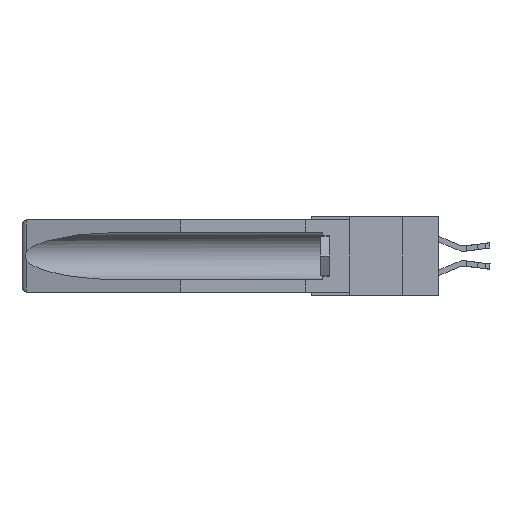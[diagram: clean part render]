
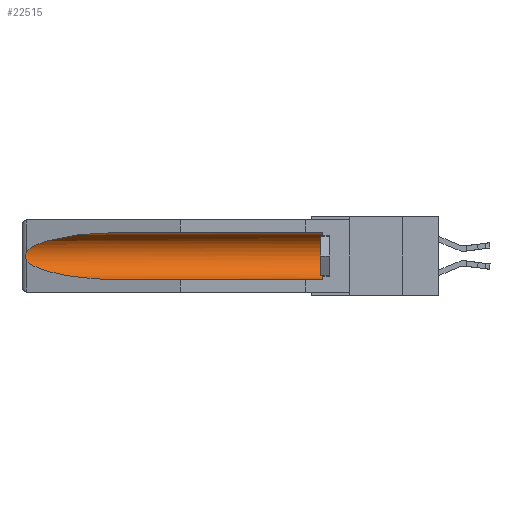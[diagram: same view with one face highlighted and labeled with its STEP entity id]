
A CAD part, left-side view. The second image highlights one B-rep face of the part: STEP entity #22515.
In plain terms, the highlighted cylindrical face has radius 2.857 mm (diameter 5.715 mm), a partial arc.
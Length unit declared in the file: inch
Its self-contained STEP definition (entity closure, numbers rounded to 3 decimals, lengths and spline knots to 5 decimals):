
#391 = CARTESIAN_POINT ( 'NONE',  ( 0.26537, 1.52718, -0.19328 ) ) ;
#412 = CARTESIAN_POINT ( 'NONE',  ( 0.155, 1.07973, -0.059 ) ) ;
#650 = ORIENTED_EDGE ( 'NONE', *, *, #18229, .T. ) ;
#932 = ORIENTED_EDGE ( 'NONE', *, *, #18708, .T. ) ;
#1380 = CARTESIAN_POINT ( 'NONE',  ( 0.25451, 1.48313, -0.24835 ) ) ;
#1624 = EDGE_CURVE ( 'NONE', #8203, #10689, #21690, .T. ) ;
#2070 = CARTESIAN_POINT ( 'NONE',  ( 0.26537, 1.52718, -0.14972 ) ) ;
#3521 = CIRCLE ( 'NONE', #14545, 0.1125 ) ;
#4706 = DIRECTION ( 'NONE',  ( 0., 1., 0. ) ) ;
#4957 = CARTESIAN_POINT ( 'NONE',  ( 0.155, 1.07973, -0.059 ) ) ;
#5436 = CARTESIAN_POINT ( 'NONE',  ( 0.2675, 1.53308, -0.16763 ) ) ;
#6120 = DIRECTION ( 'NONE',  ( 0., 1., 0. ) ) ;
#6589 = CARTESIAN_POINT ( 'NONE',  ( 0.155, 1.07973, -0.284 ) ) ;
#6967 = CARTESIAN_POINT ( 'NONE',  ( 0.2675, 1.53308, -0.17534 ) ) ;
#7113 = CARTESIAN_POINT ( 'NONE',  ( 0.26655, 1.53094, -0.18657 ) ) ;
#7624 = DIRECTION ( 'NONE',  ( 0., 0., 1. ) ) ;
#7656 = B_SPLINE_CURVE_WITH_KNOTS ( 'NONE', 3,
 ( #19102, #15642, #17405, #12399, #5436, #6967, #8620, #7113, #12183, #13880 ),
 .UNSPECIFIED., .F., .F.,
 ( 4, 2, 2, 2, 4 ),
 ( 0., 0.00029, 0.00058, 0.00087, 0.00117 ),
 .UNSPECIFIED. ) ;
#8203 = VERTEX_POINT ( 'NONE', #14624 ) ;
#8305 = CARTESIAN_POINT ( 'NONE',  ( 0.155, 1.07973, -0.284 ) ) ;
#8620 = CARTESIAN_POINT ( 'NONE',  ( 0.2673, 1.53269, -0.17917 ) ) ;
#8873 = CYLINDRICAL_SURFACE ( 'NONE', #9598, 0.1125 ) ;
#9003 = VERTEX_POINT ( 'NONE', #391 ) ;
#9062 = ORIENTED_EDGE ( 'NONE', *, *, #21922, .T. ) ;
#9598 = AXIS2_PLACEMENT_3D ( 'NONE', #14553, #10896, #7624 ) ;
#9942 = CARTESIAN_POINT ( 'NONE',  ( 0.155, -0.30754, -0.059 ) ) ;
#10052 = CARTESIAN_POINT ( 'NONE',  ( 0.25451, 1.48313, -0.09465 ) ) ;
#10334 = DIRECTION ( 'NONE',  ( 0., 0., 1. ) ) ;
#10689 = VERTEX_POINT ( 'NONE', #6589 ) ;
#10896 = DIRECTION ( 'NONE',  ( 0., 1., 0. ) ) ;
#11563 = CARTESIAN_POINT ( 'NONE',  ( 0.21114, 1.30732, -0.284 ) ) ;
#11685 = ORIENTED_EDGE ( 'NONE', *, *, #21661, .T. ) ;
#11702 = CARTESIAN_POINT ( 'NONE',  ( 0.26537, 1.52718, -0.19328 ) ) ;
#12183 = CARTESIAN_POINT ( 'NONE',  ( 0.26597, 1.5296, -0.19026 ) ) ;
#12399 = CARTESIAN_POINT ( 'NONE',  ( 0.2673, 1.5327, -0.16383 ) ) ;
#12922 = CARTESIAN_POINT ( 'NONE',  ( 0.155, -0.30754, -0.284 ) ) ;
#13310 = EDGE_CURVE ( 'NONE', #8203, #20683, #3521, .T. ) ;
#13880 = CARTESIAN_POINT ( 'NONE',  ( 0.26537, 1.52718, -0.19328 ) ) ;
#14545 = AXIS2_PLACEMENT_3D ( 'NONE', #22470, #15451, #10334 ) ;
#14553 = CARTESIAN_POINT ( 'NONE',  ( 0.155, -0.30754, -0.1715 ) ) ;
#14624 = CARTESIAN_POINT ( 'NONE',  ( 0.155, 0.126, -0.284 ) ) ;
#15451 = DIRECTION ( 'NONE',  ( 0., -1., 0. ) ) ;
#15622 = ORIENTED_EDGE ( 'NONE', *, *, #13310, .T. ) ;
#15642 = CARTESIAN_POINT ( 'NONE',  ( 0.26597, 1.52961, -0.15275 ) ) ;
#16323 = EDGE_LOOP ( 'NONE', ( #932, #650, #11685, #22556, #15622, #9062 ) ) ;
#16462 = VERTEX_POINT ( 'NONE', #2070 ) ;
#16536 = LINE ( 'NONE', #9942, #18746 ) ;
#17174 = CARTESIAN_POINT ( 'NONE',  ( 0.26537, 1.52718, -0.14972 ) ) ;
#17405 = CARTESIAN_POINT ( 'NONE',  ( 0.26654, 1.53092, -0.15636 ) ) ;
#17438 =( BOUNDED_CURVE ( )  B_SPLINE_CURVE ( 3, ( #11702, #1380, #11563, #8305 ),
 .UNSPECIFIED., .F., .F. ) 
 B_SPLINE_CURVE_WITH_KNOTS ( ( 4, 4 ),
 ( 0.1948, 1.5708 ),
 .UNSPECIFIED. ) 
 CURVE ( )  GEOMETRIC_REPRESENTATION_ITEM ( )  RATIONAL_B_SPLINE_CURVE ( ( 1., 0.848, 0.848, 1. ) ) 
 REPRESENTATION_ITEM ( '' )  );
#17898 = FACE_OUTER_BOUND ( 'NONE', #16323, .T. ) ;
#17938 = VERTEX_POINT ( 'NONE', #412 ) ;
#18229 = EDGE_CURVE ( 'NONE', #16462, #9003, #7656, .T. ) ;
#18418 = VECTOR ( 'NONE', #6120, 39.37008 ) ;
#18708 = EDGE_CURVE ( 'NONE', #17938, #16462, #19136, .T. ) ;
#18746 = VECTOR ( 'NONE', #4706, 39.37008 ) ;
#19102 = CARTESIAN_POINT ( 'NONE',  ( 0.26537, 1.52718, -0.14972 ) ) ;
#19136 =( BOUNDED_CURVE ( )  B_SPLINE_CURVE ( 3, ( #4957, #20525, #10052, #17174 ),
 .UNSPECIFIED., .F., .T. ) 
 B_SPLINE_CURVE_WITH_KNOTS ( ( 4, 4 ),
 ( 4.71239, 6.08839 ),
 .UNSPECIFIED. ) 
 CURVE ( )  GEOMETRIC_REPRESENTATION_ITEM ( )  RATIONAL_B_SPLINE_CURVE ( ( 1., 0.848, 0.848, 1. ) ) 
 REPRESENTATION_ITEM ( '' )  );
#20525 = CARTESIAN_POINT ( 'NONE',  ( 0.21114, 1.30732, -0.059 ) ) ;
#20683 = VERTEX_POINT ( 'NONE', #22003 ) ;
#21661 = EDGE_CURVE ( 'NONE', #9003, #10689, #17438, .T. ) ;
#21690 = LINE ( 'NONE', #12922, #18418 ) ;
#21922 = EDGE_CURVE ( 'NONE', #20683, #17938, #16536, .T. ) ;
#22003 = CARTESIAN_POINT ( 'NONE',  ( 0.155, 0.126, -0.059 ) ) ;
#22470 = CARTESIAN_POINT ( 'NONE',  ( 0.155, 0.126, -0.1715 ) ) ;
#22515 = ADVANCED_FACE ( 'NONE', ( #17898 ), #8873, .F. ) ;
#22556 = ORIENTED_EDGE ( 'NONE', *, *, #1624, .F. ) ;
